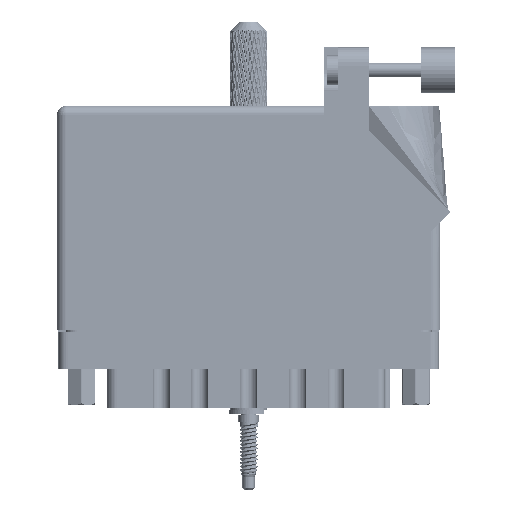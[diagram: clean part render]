
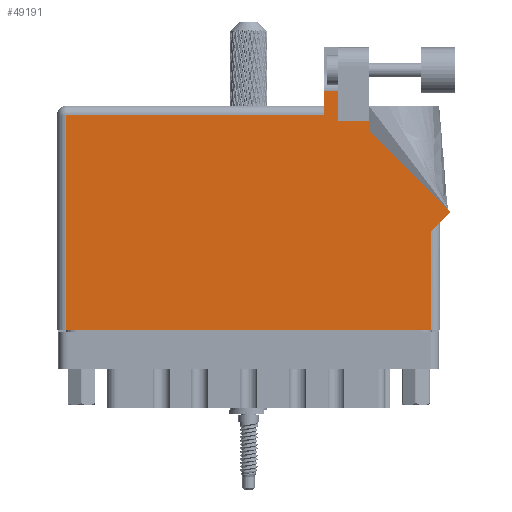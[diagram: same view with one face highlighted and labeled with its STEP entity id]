
A CAD part, front view. The second image highlights one B-rep face of the part: STEP entity #49191.
In plain terms, the highlighted face is planar.
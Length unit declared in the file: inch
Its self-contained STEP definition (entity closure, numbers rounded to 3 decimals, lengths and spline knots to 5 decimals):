
#903 = CARTESIAN_POINT ( 'NONE',  ( 2.126, 1.43, 0. ) ) ;
#4961 = LINE ( 'NONE', #123827, #84859 ) ;
#7539 = DIRECTION ( 'NONE',  ( -0.707, 0.707, 0. ) ) ;
#8091 = LINE ( 'NONE', #47749, #81464 ) ;
#10048 = LINE ( 'NONE', #60694, #21397 ) ;
#12726 = EDGE_CURVE ( 'NONE', #61552, #64917, #87831, .T. ) ;
#13369 = EDGE_LOOP ( 'NONE', ( #70405, #13936, #65222, #107245, #22135, #80666, #107429, #116196, #92593, #16639, #118498 ) ) ;
#13936 = ORIENTED_EDGE ( 'NONE', *, *, #73862, .T. ) ;
#15841 = VECTOR ( 'NONE', #91279, 39.37008 ) ;
#16639 = ORIENTED_EDGE ( 'NONE', *, *, #125645, .T. ) ;
#17060 = CARTESIAN_POINT ( 'NONE',  ( 2.612, 0.737, 0. ) ) ;
#17772 = VECTOR ( 'NONE', #7539, 39.37008 ) ;
#21397 = VECTOR ( 'NONE', #60056, 39.37008 ) ;
#22110 = EDGE_CURVE ( 'NONE', #102032, #103458, #83333, .T. ) ;
#22135 = ORIENTED_EDGE ( 'NONE', *, *, #128281, .T. ) ;
#27876 = DIRECTION ( 'NONE',  ( -1., 0., 0. ) ) ;
#28681 = VECTOR ( 'NONE', #39808, 39.37008 ) ;
#37540 = VERTEX_POINT ( 'NONE', #128397 ) ;
#39808 = DIRECTION ( 'NONE',  ( 0.707, 0.707, 0. ) ) ;
#40050 = VERTEX_POINT ( 'NONE', #903 ) ;
#41976 = CARTESIAN_POINT ( 'NONE',  ( 0., 1.53, 0. ) ) ;
#42426 = CARTESIAN_POINT ( 'NONE',  ( 2.55, 0., 0. ) ) ;
#42621 = DIRECTION ( 'NONE',  ( 0., 0., -1. ) ) ;
#42892 = VERTEX_POINT ( 'NONE', #69343 ) ;
#43161 = LINE ( 'NONE', #89923, #74833 ) ;
#44440 = LINE ( 'NONE', #124274, #81049 ) ;
#44567 = VERTEX_POINT ( 'NONE', #42426 ) ;
#45075 = CARTESIAN_POINT ( 'NONE',  ( 1.913, 1.43, 0. ) ) ;
#45912 = DIRECTION ( 'NONE',  ( 0., 1., 0. ) ) ;
#47400 = CARTESIAN_POINT ( 'NONE',  ( 2.126, 1.43, 0. ) ) ;
#47749 = CARTESIAN_POINT ( 'NONE',  ( 0., 0., 0. ) ) ;
#48396 = CARTESIAN_POINT ( 'NONE',  ( 1.913, 1.6315, 0. ) ) ;
#49191 = ADVANCED_FACE ( 'NONE', ( #51710 ), #70537, .F. ) ;
#51710 = FACE_OUTER_BOUND ( 'NONE', #13369, .T. ) ;
#52318 = CARTESIAN_POINT ( 'NONE',  ( 1.819, 1.468, 0. ) ) ;
#54135 = EDGE_CURVE ( 'NONE', #42892, #99355, #62690, .T. ) ;
#55455 = DIRECTION ( 'NONE',  ( -1., 0., 0. ) ) ;
#57234 = CARTESIAN_POINT ( 'NONE',  ( 2.55, 0.737, 0. ) ) ;
#57857 = DIRECTION ( 'NONE',  ( 0., 1., 0. ) ) ;
#59793 = CARTESIAN_POINT ( 'NONE',  ( 2.68271, 0.80771, 0. ) ) ;
#60056 = DIRECTION ( 'NONE',  ( -1., 0., 0. ) ) ;
#60515 = VECTOR ( 'NONE', #122991, 39.37008 ) ;
#60694 = CARTESIAN_POINT ( 'NONE',  ( 2.24377, 1.6315, 0. ) ) ;
#60949 = VERTEX_POINT ( 'NONE', #66189 ) ;
#61552 = VERTEX_POINT ( 'NONE', #92860 ) ;
#61569 = EDGE_CURVE ( 'NONE', #40050, #102032, #116865, .T. ) ;
#62690 = LINE ( 'NONE', #101028, #15841 ) ;
#64917 = VERTEX_POINT ( 'NONE', #59793 ) ;
#65222 = ORIENTED_EDGE ( 'NONE', *, *, #54135, .T. ) ;
#66189 = CARTESIAN_POINT ( 'NONE',  ( 0.062, 0., 0. ) ) ;
#69343 = CARTESIAN_POINT ( 'NONE',  ( 1.819, 1.6315, 0. ) ) ;
#70405 = ORIENTED_EDGE ( 'NONE', *, *, #22110, .T. ) ;
#70537 = PLANE ( 'NONE',  #88167 ) ;
#72890 = EDGE_CURVE ( 'NONE', #60949, #44567, #8091, .T. ) ;
#73081 = DIRECTION ( 'NONE',  ( -1., 0., 0. ) ) ;
#73862 = EDGE_CURVE ( 'NONE', #103458, #42892, #10048, .T. ) ;
#74833 = VECTOR ( 'NONE', #111370, 39.37008 ) ;
#77007 = LINE ( 'NONE', #96510, #17772 ) ;
#78424 = EDGE_CURVE ( 'NONE', #64917, #95101, #77007, .T. ) ;
#80666 = ORIENTED_EDGE ( 'NONE', *, *, #72890, .T. ) ;
#81049 = VECTOR ( 'NONE', #55455, 39.37008 ) ;
#81464 = VECTOR ( 'NONE', #96429, 39.37008 ) ;
#83333 = LINE ( 'NONE', #45075, #60515 ) ;
#84859 = VECTOR ( 'NONE', #45912, 39.37008 ) ;
#87831 = LINE ( 'NONE', #17060, #28681 ) ;
#88167 = AXIS2_PLACEMENT_3D ( 'NONE', #41976, #42621, #73081 ) ;
#89923 = CARTESIAN_POINT ( 'NONE',  ( 0.062, 0., 0. ) ) ;
#91279 = DIRECTION ( 'NONE',  ( 0., -1., 0. ) ) ;
#92593 = ORIENTED_EDGE ( 'NONE', *, *, #78424, .T. ) ;
#92860 = CARTESIAN_POINT ( 'NONE',  ( 2.55, 0.675, 0. ) ) ;
#95101 = VERTEX_POINT ( 'NONE', #126123 ) ;
#96429 = DIRECTION ( 'NONE',  ( 1., 0., 0. ) ) ;
#96510 = CARTESIAN_POINT ( 'NONE',  ( 2.68271, 0.80771, 0. ) ) ;
#99355 = VERTEX_POINT ( 'NONE', #52318 ) ;
#101028 = CARTESIAN_POINT ( 'NONE',  ( 1.819, 1.53, 0. ) ) ;
#102032 = VERTEX_POINT ( 'NONE', #114143 ) ;
#103458 = VERTEX_POINT ( 'NONE', #48396 ) ;
#107245 = ORIENTED_EDGE ( 'NONE', *, *, #128311, .T. ) ;
#107429 = ORIENTED_EDGE ( 'NONE', *, *, #125365, .T. ) ;
#111370 = DIRECTION ( 'NONE',  ( 0., -1., 0. ) ) ;
#114143 = CARTESIAN_POINT ( 'NONE',  ( 1.913, 1.43, 0. ) ) ;
#116196 = ORIENTED_EDGE ( 'NONE', *, *, #12726, .T. ) ;
#116865 = LINE ( 'NONE', #47400, #118063 ) ;
#118063 = VECTOR ( 'NONE', #27876, 39.37008 ) ;
#118498 = ORIENTED_EDGE ( 'NONE', *, *, #61569, .T. ) ;
#122991 = DIRECTION ( 'NONE',  ( 0., 1., 0. ) ) ;
#123827 = CARTESIAN_POINT ( 'NONE',  ( 2.126, 1.36442, 0. ) ) ;
#124274 = CARTESIAN_POINT ( 'NONE',  ( 0., 1.468, 0. ) ) ;
#124774 = LINE ( 'NONE', #57234, #128468 ) ;
#125365 = EDGE_CURVE ( 'NONE', #44567, #61552, #124774, .T. ) ;
#125645 = EDGE_CURVE ( 'NONE', #95101, #40050, #4961, .T. ) ;
#126123 = CARTESIAN_POINT ( 'NONE',  ( 2.126, 1.36442, 0. ) ) ;
#128281 = EDGE_CURVE ( 'NONE', #37540, #60949, #43161, .T. ) ;
#128311 = EDGE_CURVE ( 'NONE', #99355, #37540, #44440, .T. ) ;
#128397 = CARTESIAN_POINT ( 'NONE',  ( 0.062, 1.468, 0. ) ) ;
#128468 = VECTOR ( 'NONE', #57857, 39.37008 ) ;
